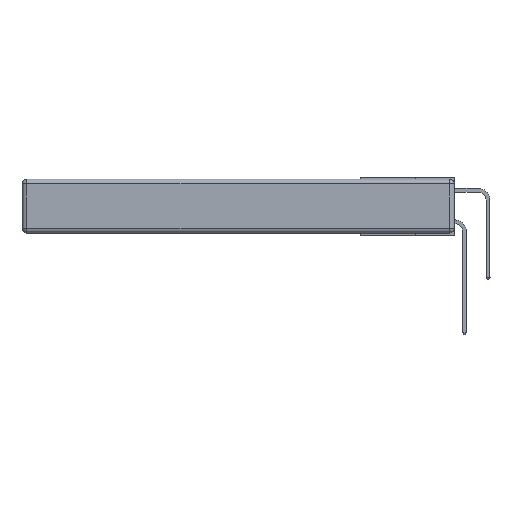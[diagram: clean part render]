
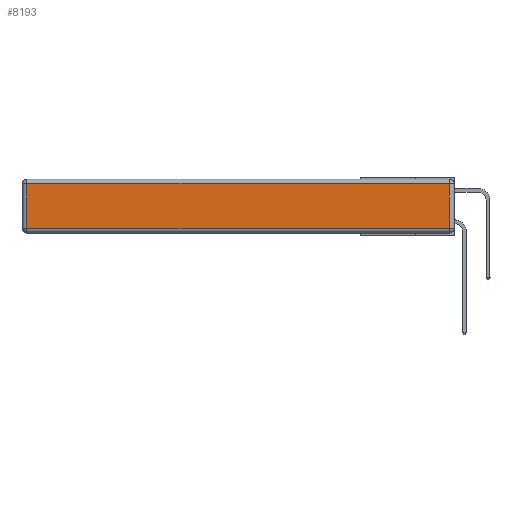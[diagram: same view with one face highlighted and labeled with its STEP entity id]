
A CAD part, left-side view. The second image highlights one B-rep face of the part: STEP entity #8193.
In plain terms, the highlighted planar face has unit normal (-1, 0, 0).
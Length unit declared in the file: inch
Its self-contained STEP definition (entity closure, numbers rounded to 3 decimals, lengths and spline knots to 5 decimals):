
#1378 = VECTOR ( 'NONE', #2834, 39.37008 ) ;
#1417 = CARTESIAN_POINT ( 'NONE',  ( 0., 0., -0.343 ) ) ;
#2059 = FACE_OUTER_BOUND ( 'NONE', #13012, .T. ) ;
#2672 = EDGE_CURVE ( 'NONE', #6142, #7182, #3184, .T. ) ;
#2834 = DIRECTION ( 'NONE',  ( 0., -1., 0. ) ) ;
#3184 = LINE ( 'NONE', #14080, #6372 ) ;
#3397 = ORIENTED_EDGE ( 'NONE', *, *, #15007, .T. ) ;
#3586 = VECTOR ( 'NONE', #15591, 39.37008 ) ;
#4193 = CARTESIAN_POINT ( 'NONE',  ( 0., 2.72, -0.343 ) ) ;
#4952 = ORIENTED_EDGE ( 'NONE', *, *, #12212, .T. ) ;
#5495 = AXIS2_PLACEMENT_3D ( 'NONE', #1417, #12690, #10282 ) ;
#6142 = VERTEX_POINT ( 'NONE', #11484 ) ;
#6372 = VECTOR ( 'NONE', #6493, 39.37008 ) ;
#6493 = DIRECTION ( 'NONE',  ( 0., 1., 0. ) ) ;
#7182 = VERTEX_POINT ( 'NONE', #8194 ) ;
#7746 = LINE ( 'NONE', #4193, #3586 ) ;
#8193 = ADVANCED_FACE ( 'NONE', ( #2059 ), #16383, .T. ) ;
#8194 = CARTESIAN_POINT ( 'NONE',  ( 0., 2.72, -0.03 ) ) ;
#9205 = CARTESIAN_POINT ( 'NONE',  ( 0., 2.72, -0.313 ) ) ;
#9905 = VECTOR ( 'NONE', #10528, 39.37008 ) ;
#10070 = CARTESIAN_POINT ( 'NONE',  ( 0., 0., -0.313 ) ) ;
#10282 = DIRECTION ( 'NONE',  ( 0., 0., 1. ) ) ;
#10330 = EDGE_CURVE ( 'NONE', #15130, #11931, #13677, .T. ) ;
#10528 = DIRECTION ( 'NONE',  ( 0., 0., 1. ) ) ;
#11484 = CARTESIAN_POINT ( 'NONE',  ( 0., 0.03, -0.03 ) ) ;
#11931 = VERTEX_POINT ( 'NONE', #12614 ) ;
#12212 = EDGE_CURVE ( 'NONE', #7182, #15130, #7746, .T. ) ;
#12614 = CARTESIAN_POINT ( 'NONE',  ( 0., 0.03, -0.313 ) ) ;
#12690 = DIRECTION ( 'NONE',  ( -1., 0., 0. ) ) ;
#13012 = EDGE_LOOP ( 'NONE', ( #15981, #3397, #13679, #4952 ) ) ;
#13488 = LINE ( 'NONE', #15637, #9905 ) ;
#13677 = LINE ( 'NONE', #10070, #1378 ) ;
#13679 = ORIENTED_EDGE ( 'NONE', *, *, #2672, .T. ) ;
#14080 = CARTESIAN_POINT ( 'NONE',  ( 0., 2.75, -0.03 ) ) ;
#15007 = EDGE_CURVE ( 'NONE', #11931, #6142, #13488, .T. ) ;
#15130 = VERTEX_POINT ( 'NONE', #9205 ) ;
#15591 = DIRECTION ( 'NONE',  ( 0., 0., -1. ) ) ;
#15637 = CARTESIAN_POINT ( 'NONE',  ( 0., 0.03, -0.343 ) ) ;
#15981 = ORIENTED_EDGE ( 'NONE', *, *, #10330, .T. ) ;
#16383 = PLANE ( 'NONE',  #5495 ) ;
